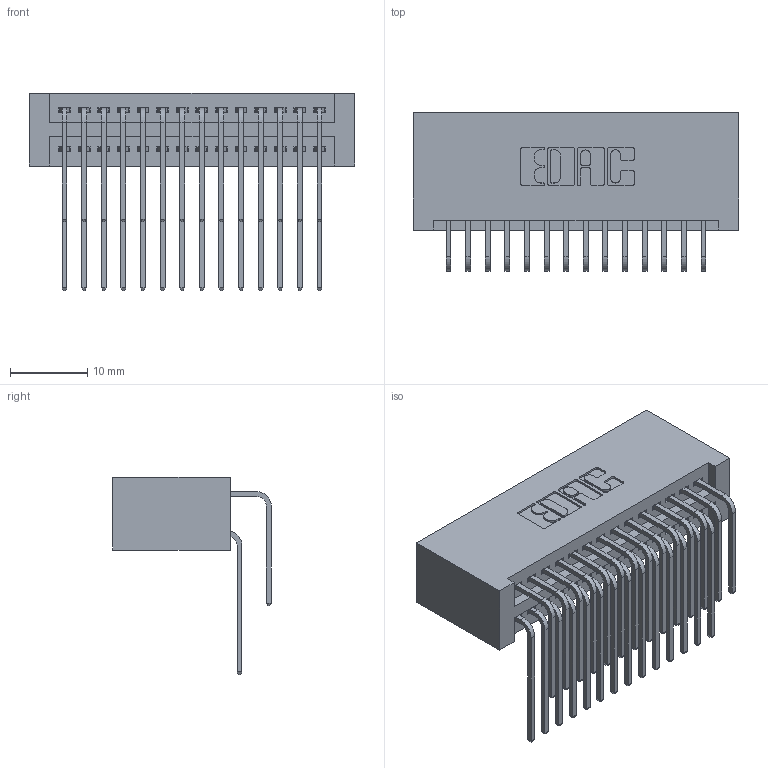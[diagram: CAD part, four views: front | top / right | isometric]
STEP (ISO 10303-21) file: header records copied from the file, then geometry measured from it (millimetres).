
FILE_DESCRIPTION (( 'STEP AP203' ), '1' );
FILE_NAME ('395-028-559-201.STEP', '2018-11-10T15:47:41', ( '' ), ( '' ), 'SwSTEP 2.0', 'SolidWorks 2016', '' );
FILE_SCHEMA (( 'CONFIG_CONTROL_DESIGN' ));
Length unit declared in the file: inch
Products named in the file (4): 345-292-001_558 559 Tail - 1; 395-028-559-201; 345-292-001_559 Tail - 2; 345 Part_No Mounting Lugs
Assembly tree (29 placements, depth 2):
  395-028-559-201
    345 Part_No Mounting Lugs
    345-292-001_558 559 Tail - 1  x14
    345-292-001_559 Tail - 2  x14
Bounding box: 42.16 x 20.56 x 25.53 mm (x, y, z)
Volume: 4613.4 mm3; surface area: 7339.9 mm2
Topology: 29 solids, 29 shells, 1574 faces, 4657 edges, 3066 vertices
Faces by surface type: plane 1056, cylinder 518
Entity records: 16129 total; most frequent: CARTESIAN_POINT 2775, ORIENTED_EDGE 2658, DIRECTION 2449, EDGE_CURVE 1329, VECTOR 1109, LINE 1109, VERTEX_POINT 882, AXIS2_PLACEMENT_3D 670
